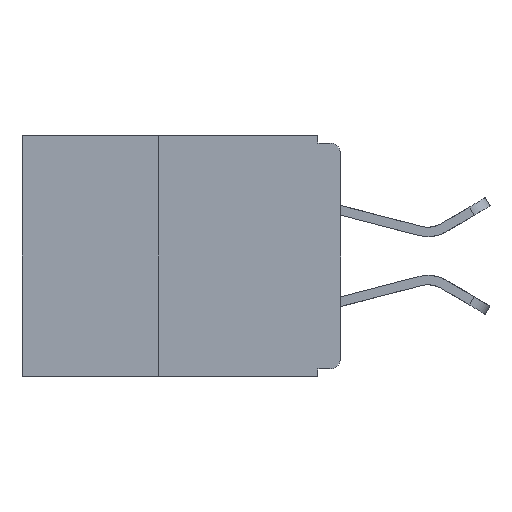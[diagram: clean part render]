
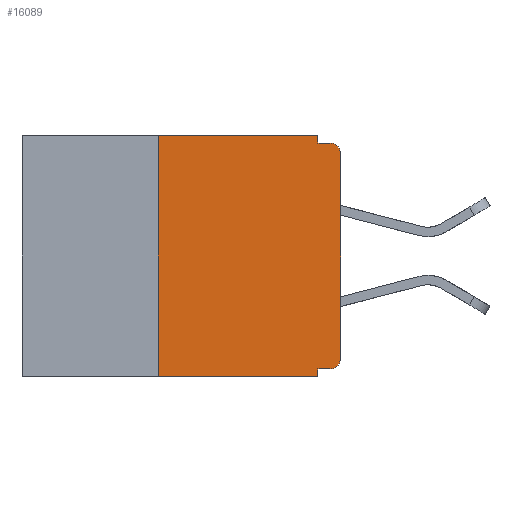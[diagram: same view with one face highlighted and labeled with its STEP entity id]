
A CAD part, left-side view. The second image highlights one B-rep face of the part: STEP entity #16089.
In plain terms, the highlighted planar face has unit normal (-1, 0, 0).
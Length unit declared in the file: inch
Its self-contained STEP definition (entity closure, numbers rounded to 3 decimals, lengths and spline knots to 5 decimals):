
#613 = VERTEX_POINT ( 'NONE', #14293 ) ;
#720 = VERTEX_POINT ( 'NONE', #7227 ) ;
#1178 = DIRECTION ( 'NONE',  ( 0., -1., 0. ) ) ;
#1891 = VECTOR ( 'NONE', #22410, 39.37008 ) ;
#2060 = VERTEX_POINT ( 'NONE', #23115 ) ;
#2155 = LINE ( 'NONE', #24916, #21151 ) ;
#2271 = ORIENTED_EDGE ( 'NONE', *, *, #21649, .T. ) ;
#2582 = LINE ( 'NONE', #20298, #1891 ) ;
#3309 = CARTESIAN_POINT ( 'NONE',  ( 0., 0.25, -0.33 ) ) ;
#3431 = CARTESIAN_POINT ( 'NONE',  ( 0., 0.437, -0.33 ) ) ;
#3468 = LINE ( 'NONE', #3431, #14299 ) ;
#3936 = CARTESIAN_POINT ( 'NONE',  ( 0., 0.015, -0.025 ) ) ;
#4700 = ORIENTED_EDGE ( 'NONE', *, *, #19527, .T. ) ;
#5018 = ORIENTED_EDGE ( 'NONE', *, *, #15506, .F. ) ;
#5471 = CARTESIAN_POINT ( 'NONE',  ( 0., 0., -0.025 ) ) ;
#5889 = VECTOR ( 'NONE', #25592, 39.37008 ) ;
#6116 = DIRECTION ( 'NONE',  ( 0., 0., -1. ) ) ;
#6240 = AXIS2_PLACEMENT_3D ( 'NONE', #21805, #9082, #23891 ) ;
#6730 = ORIENTED_EDGE ( 'NONE', *, *, #6835, .F. ) ;
#6835 = EDGE_CURVE ( 'NONE', #10627, #18349, #8816, .T. ) ;
#7060 = CARTESIAN_POINT ( 'NONE',  ( 0., 0.031, -0.33 ) ) ;
#7227 = CARTESIAN_POINT ( 'NONE',  ( 0., 0.031, -0.01 ) ) ;
#7961 = DIRECTION ( 'NONE',  ( -1., 0., 0. ) ) ;
#8735 = DIRECTION ( 'NONE',  ( 0., -1., 0. ) ) ;
#8816 = LINE ( 'NONE', #16728, #25019 ) ;
#8916 = CIRCLE ( 'NONE', #12236, 0.015 ) ;
#9082 = DIRECTION ( 'NONE',  ( 1., 0., 0. ) ) ;
#9446 = FACE_OUTER_BOUND ( 'NONE', #27050, .T. ) ;
#9869 = DIRECTION ( 'NONE',  ( 0., 0., 1. ) ) ;
#10627 = VERTEX_POINT ( 'NONE', #19139 ) ;
#11120 = VECTOR ( 'NONE', #22013, 39.37008 ) ;
#11402 = AXIS2_PLACEMENT_3D ( 'NONE', #20679, #7961, #22793 ) ;
#11461 = CARTESIAN_POINT ( 'NONE',  ( 0., 0., -0.01 ) ) ;
#11665 = VERTEX_POINT ( 'NONE', #11725 ) ;
#11725 = CARTESIAN_POINT ( 'NONE',  ( 0., 0.015, -0.01 ) ) ;
#12236 = AXIS2_PLACEMENT_3D ( 'NONE', #3936, #18975, #6116 ) ;
#12328 = LINE ( 'NONE', #23544, #5889 ) ;
#13111 = ORIENTED_EDGE ( 'NONE', *, *, #26622, .T. ) ;
#13315 = PLANE ( 'NONE',  #6240 ) ;
#13468 = ORIENTED_EDGE ( 'NONE', *, *, #17919, .F. ) ;
#13472 = VERTEX_POINT ( 'NONE', #5471 ) ;
#13636 = CIRCLE ( 'NONE', #11402, 0.015 ) ;
#14293 = CARTESIAN_POINT ( 'NONE',  ( 0., 0.031, 0. ) ) ;
#14299 = VECTOR ( 'NONE', #1178, 39.37008 ) ;
#14679 = VECTOR ( 'NONE', #9869, 39.37008 ) ;
#14812 = ORIENTED_EDGE ( 'NONE', *, *, #20925, .F. ) ;
#15129 = CARTESIAN_POINT ( 'NONE',  ( 0., 0.437, 0. ) ) ;
#15354 = LINE ( 'NONE', #3309, #14679 ) ;
#15506 = EDGE_CURVE ( 'NONE', #720, #11665, #17466, .T. ) ;
#15657 = CARTESIAN_POINT ( 'NONE',  ( 0., 0.25, -0.33 ) ) ;
#16055 = VECTOR ( 'NONE', #8735, 39.37008 ) ;
#16089 = ADVANCED_FACE ( 'NONE', ( #9446 ), #13315, .F. ) ;
#16728 = CARTESIAN_POINT ( 'NONE',  ( 0., 0., -0.32 ) ) ;
#16732 = LINE ( 'NONE', #15129, #16055 ) ;
#16733 = EDGE_CURVE ( 'NONE', #18349, #27427, #2582, .T. ) ;
#17132 = ORIENTED_EDGE ( 'NONE', *, *, #26437, .F. ) ;
#17430 = VERTEX_POINT ( 'NONE', #18367 ) ;
#17466 = LINE ( 'NONE', #11461, #11120 ) ;
#17919 = EDGE_CURVE ( 'NONE', #17430, #613, #16732, .T. ) ;
#18349 = VERTEX_POINT ( 'NONE', #24894 ) ;
#18367 = CARTESIAN_POINT ( 'NONE',  ( 0., 0.25, 0. ) ) ;
#18851 = DIRECTION ( 'NONE',  ( 0., 1., 0. ) ) ;
#18975 = DIRECTION ( 'NONE',  ( -1., 0., 0. ) ) ;
#19139 = CARTESIAN_POINT ( 'NONE',  ( 0., 0.015, -0.32 ) ) ;
#19527 = EDGE_CURVE ( 'NONE', #20448, #27427, #3468, .T. ) ;
#20298 = CARTESIAN_POINT ( 'NONE',  ( 0., 0.031, -0.33 ) ) ;
#20448 = VERTEX_POINT ( 'NONE', #15657 ) ;
#20679 = CARTESIAN_POINT ( 'NONE',  ( 0., 0.015, -0.305 ) ) ;
#20925 = EDGE_CURVE ( 'NONE', #20448, #17430, #15354, .T. ) ;
#21151 = VECTOR ( 'NONE', #26927, 39.37008 ) ;
#21649 = EDGE_CURVE ( 'NONE', #10627, #2060, #13636, .T. ) ;
#21805 = CARTESIAN_POINT ( 'NONE',  ( 0., 0.437, 0. ) ) ;
#22013 = DIRECTION ( 'NONE',  ( 0., -1., 0. ) ) ;
#22380 = ORIENTED_EDGE ( 'NONE', *, *, #16733, .F. ) ;
#22410 = DIRECTION ( 'NONE',  ( 0., 0., -1. ) ) ;
#22793 = DIRECTION ( 'NONE',  ( 0., 0., -1. ) ) ;
#23115 = CARTESIAN_POINT ( 'NONE',  ( 0., 0., -0.305 ) ) ;
#23544 = CARTESIAN_POINT ( 'NONE',  ( 0., 0., 0. ) ) ;
#23891 = DIRECTION ( 'NONE',  ( 0., 0., -1. ) ) ;
#24894 = CARTESIAN_POINT ( 'NONE',  ( 0., 0.031, -0.32 ) ) ;
#24916 = CARTESIAN_POINT ( 'NONE',  ( 0., 0.031, 0. ) ) ;
#24955 = ORIENTED_EDGE ( 'NONE', *, *, #27143, .T. ) ;
#25019 = VECTOR ( 'NONE', #18851, 39.37008 ) ;
#25592 = DIRECTION ( 'NONE',  ( 0., 0., 1. ) ) ;
#26437 = EDGE_CURVE ( 'NONE', #613, #720, #2155, .T. ) ;
#26622 = EDGE_CURVE ( 'NONE', #2060, #13472, #12328, .T. ) ;
#26927 = DIRECTION ( 'NONE',  ( 0., 0., -1. ) ) ;
#27050 = EDGE_LOOP ( 'NONE', ( #13111, #24955, #5018, #17132, #13468, #14812, #4700, #22380, #6730, #2271 ) ) ;
#27143 = EDGE_CURVE ( 'NONE', #13472, #11665, #8916, .T. ) ;
#27427 = VERTEX_POINT ( 'NONE', #7060 ) ;
